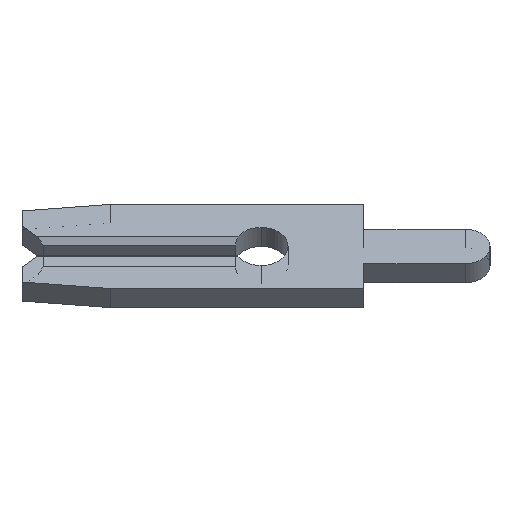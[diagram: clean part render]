
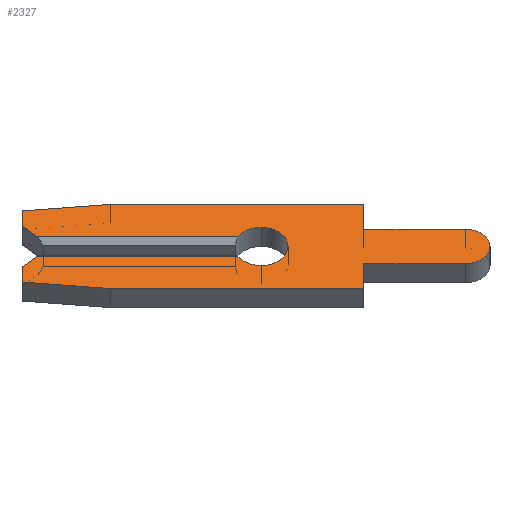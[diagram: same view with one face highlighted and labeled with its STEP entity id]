
A CAD part, left-side view. The second image highlights one B-rep face of the part: STEP entity #2327.
In plain terms, the highlighted face is planar.
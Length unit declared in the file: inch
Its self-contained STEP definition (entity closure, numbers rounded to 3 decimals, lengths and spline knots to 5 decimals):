
#10 = VECTOR ( 'NONE', #955, 39.37008 ) ;
#22 = CARTESIAN_POINT ( 'NONE',  ( -0.013, 0., 0. ) ) ;
#28 = DIRECTION ( 'NONE',  ( -1., 0., 0. ) ) ;
#39 = CARTESIAN_POINT ( 'NONE',  ( -0.013, 0., -0.026 ) ) ;
#50 = AXIS2_PLACEMENT_3D ( 'NONE', #1739, #28, #216 ) ;
#61 = VECTOR ( 'NONE', #1076, 39.37008 ) ;
#63 = VERTEX_POINT ( 'NONE', #1136 ) ;
#65 = AXIS2_PLACEMENT_3D ( 'NONE', #22, #775, #1543 ) ;
#77 = CARTESIAN_POINT ( 'NONE',  ( -0.013, 0.231, -0.028 ) ) ;
#86 = LINE ( 'NONE', #916, #2049 ) ;
#89 = ORIENTED_EDGE ( 'NONE', *, *, #532, .F. ) ;
#90 = VECTOR ( 'NONE', #1419, 39.37008 ) ;
#99 = CARTESIAN_POINT ( 'NONE',  ( -0.013, -0.099, -0.0235 ) ) ;
#114 = ORIENTED_EDGE ( 'NONE', *, *, #1799, .F. ) ;
#128 = EDGE_CURVE ( 'NONE', #1299, #402, #1428, .T. ) ;
#179 = CARTESIAN_POINT ( 'NONE',  ( -0.013, 0.231, 0.028 ) ) ;
#180 = VECTOR ( 'NONE', #796, 39.37008 ) ;
#212 = EDGE_CURVE ( 'NONE', #1030, #402, #2147, .T. ) ;
#216 = DIRECTION ( 'NONE',  ( 0., 0., -1. ) ) ;
#235 = CARTESIAN_POINT ( 'NONE',  ( -0.013, 0., 0. ) ) ;
#273 = DIRECTION ( 'NONE',  ( 0., 0., -1. ) ) ;
#279 = EDGE_CURVE ( 'NONE', #764, #1765, #1220, .T. ) ;
#280 = DIRECTION ( 'NONE',  ( 1., 0., 0. ) ) ;
#350 = DIRECTION ( 'NONE',  ( 0., 0., -1. ) ) ;
#374 = EDGE_CURVE ( 'NONE', #1218, #764, #1157, .T. ) ;
#376 = FACE_OUTER_BOUND ( 'NONE', #1034, .T. ) ;
#386 = CARTESIAN_POINT ( 'NONE',  ( -0.013, 0.231, 0.013 ) ) ;
#402 = VERTEX_POINT ( 'NONE', #452 ) ;
#407 = LINE ( 'NONE', #1960, #968 ) ;
#421 = EDGE_CURVE ( 'NONE', #1765, #1608, #1303, .T. ) ;
#422 = DIRECTION ( 'NONE',  ( 0., 0., -1. ) ) ;
#445 = ORIENTED_EDGE ( 'NONE', *, *, #888, .F. ) ;
#447 = CARTESIAN_POINT ( 'NONE',  ( -0.013, -0.1975, 0. ) ) ;
#452 = CARTESIAN_POINT ( 'NONE',  ( -0.013, 0.02252, 0.013 ) ) ;
#473 = CIRCLE ( 'NONE', #50, 0.026 ) ;
#499 = CARTESIAN_POINT ( 'NONE',  ( -0.013, 0.146, 0.0575 ) ) ;
#505 = CARTESIAN_POINT ( 'NONE',  ( -0.013, 0.231, 0.028 ) ) ;
#516 = VERTEX_POINT ( 'NONE', #499 ) ;
#522 = LINE ( 'NONE', #1235, #1732 ) ;
#529 = DIRECTION ( 'NONE',  ( 0., -1., 0. ) ) ;
#532 = EDGE_CURVE ( 'NONE', #1030, #1182, #407, .T. ) ;
#545 = CARTESIAN_POINT ( 'NONE',  ( -0.013, -0.099, -0.0575 ) ) ;
#558 = VERTEX_POINT ( 'NONE', #1029 ) ;
#580 = LINE ( 'NONE', #77, #1882 ) ;
#612 = CARTESIAN_POINT ( 'NONE',  ( -0.013, -0.099, 0.0575 ) ) ;
#620 = DIRECTION ( 'NONE',  ( 0., 0., -1. ) ) ;
#623 = DIRECTION ( 'NONE',  ( 1., 0., 0. ) ) ;
#673 = ORIENTED_EDGE ( 'NONE', *, *, #1398, .F. ) ;
#676 = ORIENTED_EDGE ( 'NONE', *, *, #2408, .F. ) ;
#717 = EDGE_CURVE ( 'NONE', #2233, #1760, #1151, .T. ) ;
#756 = VECTOR ( 'NONE', #350, 39.37008 ) ;
#764 = VERTEX_POINT ( 'NONE', #1035 ) ;
#775 = DIRECTION ( 'NONE',  ( -1., 0., 0. ) ) ;
#792 = ORIENTED_EDGE ( 'NONE', *, *, #1779, .F. ) ;
#796 = DIRECTION ( 'NONE',  ( 0., -1., 0. ) ) ;
#802 = CARTESIAN_POINT ( 'NONE',  ( -0.013, 0.216, -0.013 ) ) ;
#826 = ORIENTED_EDGE ( 'NONE', *, *, #421, .F. ) ;
#829 = VECTOR ( 'NONE', #1155, 39.37008 ) ;
#832 = EDGE_CURVE ( 'NONE', #1669, #1249, #522, .T. ) ;
#888 = EDGE_CURVE ( 'NONE', #1760, #63, #1148, .T. ) ;
#897 = DIRECTION ( 'NONE',  ( 0., 0., 1. ) ) ;
#916 = CARTESIAN_POINT ( 'NONE',  ( -0.013, 0.146, 0.0575 ) ) ;
#917 = ORIENTED_EDGE ( 'NONE', *, *, #212, .T. ) ;
#951 = ORIENTED_EDGE ( 'NONE', *, *, #2044, .F. ) ;
#955 = DIRECTION ( 'NONE',  ( 0., -1., 0. ) ) ;
#968 = VECTOR ( 'NONE', #1994, 39.37008 ) ;
#976 = EDGE_CURVE ( 'NONE', #516, #1218, #86, .T. ) ;
#997 = VECTOR ( 'NONE', #1406, 39.37008 ) ;
#1008 = CARTESIAN_POINT ( 'NONE',  ( -0.013, 0.231, -0.028 ) ) ;
#1010 = DIRECTION ( 'NONE',  ( 0., 0., 1. ) ) ;
#1029 = CARTESIAN_POINT ( 'NONE',  ( -0.013, -0.099, -0.0235 ) ) ;
#1030 = VERTEX_POINT ( 'NONE', #2061 ) ;
#1034 = EDGE_LOOP ( 'NONE', ( #917, #1662, #2376, #792, #445, #1877, #951, #114, #1629, #676, #2052, #826, #2370, #2000, #2352, #1609, #673, #89 ) ) ;
#1035 = CARTESIAN_POINT ( 'NONE',  ( -0.013, -0.099, 0.0235 ) ) ;
#1061 = VERTEX_POINT ( 'NONE', #1462 ) ;
#1063 = AXIS2_PLACEMENT_3D ( 'NONE', #235, #1945, #422 ) ;
#1076 = DIRECTION ( 'NONE',  ( 0., -0.995, 0.105 ) ) ;
#1087 = VECTOR ( 'NONE', #529, 39.37008 ) ;
#1112 = AXIS2_PLACEMENT_3D ( 'NONE', #1990, #280, #620 ) ;
#1136 = CARTESIAN_POINT ( 'NONE',  ( -0.013, 0.02252, -0.013 ) ) ;
#1148 = LINE ( 'NONE', #2029, #1087 ) ;
#1151 = LINE ( 'NONE', #1453, #90 ) ;
#1155 = DIRECTION ( 'NONE',  ( 0., 0.995, 0.105 ) ) ;
#1157 = LINE ( 'NONE', #612, #1555 ) ;
#1182 = VERTEX_POINT ( 'NONE', #505 ) ;
#1185 = EDGE_CURVE ( 'NONE', #1061, #516, #1521, .T. ) ;
#1215 = CIRCLE ( 'NONE', #1063, 0.026 ) ;
#1218 = VERTEX_POINT ( 'NONE', #1719 ) ;
#1219 = CARTESIAN_POINT ( 'NONE',  ( -0.013, -0.099, 0.0235 ) ) ;
#1220 = LINE ( 'NONE', #1219, #180 ) ;
#1235 = CARTESIAN_POINT ( 'NONE',  ( -0.013, 0.146, -0.0575 ) ) ;
#1249 = VERTEX_POINT ( 'NONE', #1485 ) ;
#1269 = DIRECTION ( 'NONE',  ( 0., -1., 0. ) ) ;
#1294 = CARTESIAN_POINT ( 'NONE',  ( -0.013, 0., 0.026 ) ) ;
#1299 = VERTEX_POINT ( 'NONE', #1294 ) ;
#1303 = CIRCLE ( 'NONE', #1371, 0.0235 ) ;
#1366 = CARTESIAN_POINT ( 'NONE',  ( -0.013, 0.231, -0.04857 ) ) ;
#1371 = AXIS2_PLACEMENT_3D ( 'NONE', #447, #623, #1010 ) ;
#1398 = EDGE_CURVE ( 'NONE', #1182, #1061, #2382, .T. ) ;
#1406 = DIRECTION ( 'NONE',  ( 0., 1., 0. ) ) ;
#1419 = DIRECTION ( 'NONE',  ( 0., -0.707, 0.707 ) ) ;
#1428 = CIRCLE ( 'NONE', #65, 0.026 ) ;
#1453 = CARTESIAN_POINT ( 'NONE',  ( -0.013, 0.2105, -0.0075 ) ) ;
#1462 = CARTESIAN_POINT ( 'NONE',  ( -0.013, 0.231, 0.04857 ) ) ;
#1474 = CARTESIAN_POINT ( 'NONE',  ( -0.013, 0.231, 0.04857 ) ) ;
#1485 = CARTESIAN_POINT ( 'NONE',  ( -0.013, 0.146, -0.0575 ) ) ;
#1511 = DIRECTION ( 'NONE',  ( 0., 0., 1. ) ) ;
#1521 = LINE ( 'NONE', #1474, #61 ) ;
#1543 = DIRECTION ( 'NONE',  ( 0., 0., -1. ) ) ;
#1555 = VECTOR ( 'NONE', #273, 39.37008 ) ;
#1603 = PLANE ( 'NONE',  #1112 ) ;
#1608 = VERTEX_POINT ( 'NONE', #2277 ) ;
#1609 = ORIENTED_EDGE ( 'NONE', *, *, #1185, .F. ) ;
#1629 = ORIENTED_EDGE ( 'NONE', *, *, #832, .F. ) ;
#1662 = ORIENTED_EDGE ( 'NONE', *, *, #128, .F. ) ;
#1669 = VERTEX_POINT ( 'NONE', #545 ) ;
#1719 = CARTESIAN_POINT ( 'NONE',  ( -0.013, -0.099, 0.0575 ) ) ;
#1732 = VECTOR ( 'NONE', #2208, 39.37008 ) ;
#1739 = CARTESIAN_POINT ( 'NONE',  ( -0.013, 0., 0. ) ) ;
#1760 = VERTEX_POINT ( 'NONE', #802 ) ;
#1765 = VERTEX_POINT ( 'NONE', #1957 ) ;
#1779 = EDGE_CURVE ( 'NONE', #63, #1975, #473, .T. ) ;
#1796 = LINE ( 'NONE', #2310, #829 ) ;
#1799 = EDGE_CURVE ( 'NONE', #1249, #2080, #1796, .T. ) ;
#1827 = LINE ( 'NONE', #2041, #756 ) ;
#1855 = LINE ( 'NONE', #99, #997 ) ;
#1877 = ORIENTED_EDGE ( 'NONE', *, *, #717, .F. ) ;
#1882 = VECTOR ( 'NONE', #897, 39.37008 ) ;
#1890 = VECTOR ( 'NONE', #1511, 39.37008 ) ;
#1945 = DIRECTION ( 'NONE',  ( -1., 0., 0. ) ) ;
#1957 = CARTESIAN_POINT ( 'NONE',  ( -0.013, -0.1975, 0.0235 ) ) ;
#1960 = CARTESIAN_POINT ( 'NONE',  ( -0.013, 0.2105, 0.0075 ) ) ;
#1968 = EDGE_CURVE ( 'NONE', #1975, #1299, #1215, .T. ) ;
#1975 = VERTEX_POINT ( 'NONE', #39 ) ;
#1990 = CARTESIAN_POINT ( 'NONE',  ( -0.013, 0., 0. ) ) ;
#1994 = DIRECTION ( 'NONE',  ( 0., 0.707, 0.707 ) ) ;
#2000 = ORIENTED_EDGE ( 'NONE', *, *, #374, .F. ) ;
#2029 = CARTESIAN_POINT ( 'NONE',  ( -0.013, 0., -0.013 ) ) ;
#2041 = CARTESIAN_POINT ( 'NONE',  ( -0.013, -0.099, -0.0575 ) ) ;
#2044 = EDGE_CURVE ( 'NONE', #2080, #2233, #580, .T. ) ;
#2049 = VECTOR ( 'NONE', #1269, 39.37008 ) ;
#2052 = ORIENTED_EDGE ( 'NONE', *, *, #2281, .F. ) ;
#2061 = CARTESIAN_POINT ( 'NONE',  ( -0.013, 0.216, 0.013 ) ) ;
#2080 = VERTEX_POINT ( 'NONE', #1366 ) ;
#2147 = LINE ( 'NONE', #386, #10 ) ;
#2208 = DIRECTION ( 'NONE',  ( 0., 1., 0. ) ) ;
#2233 = VERTEX_POINT ( 'NONE', #1008 ) ;
#2277 = CARTESIAN_POINT ( 'NONE',  ( -0.013, -0.1975, -0.0235 ) ) ;
#2281 = EDGE_CURVE ( 'NONE', #1608, #558, #1855, .T. ) ;
#2310 = CARTESIAN_POINT ( 'NONE',  ( -0.013, 0.231, -0.04857 ) ) ;
#2327 = ADVANCED_FACE ( 'NONE', ( #376 ), #1603, .F. ) ;
#2352 = ORIENTED_EDGE ( 'NONE', *, *, #976, .F. ) ;
#2370 = ORIENTED_EDGE ( 'NONE', *, *, #279, .F. ) ;
#2376 = ORIENTED_EDGE ( 'NONE', *, *, #1968, .F. ) ;
#2382 = LINE ( 'NONE', #179, #1890 ) ;
#2408 = EDGE_CURVE ( 'NONE', #558, #1669, #1827, .T. ) ;
